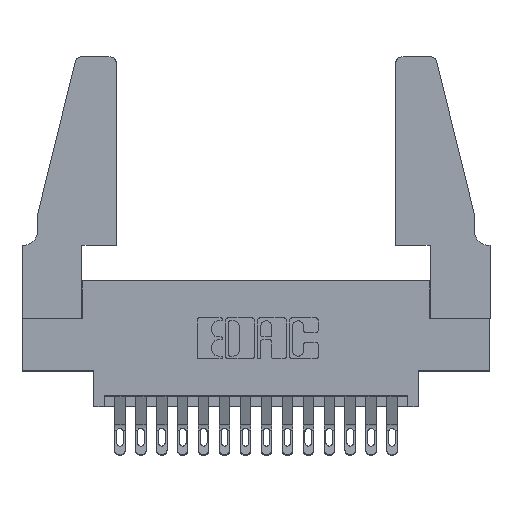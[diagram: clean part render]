
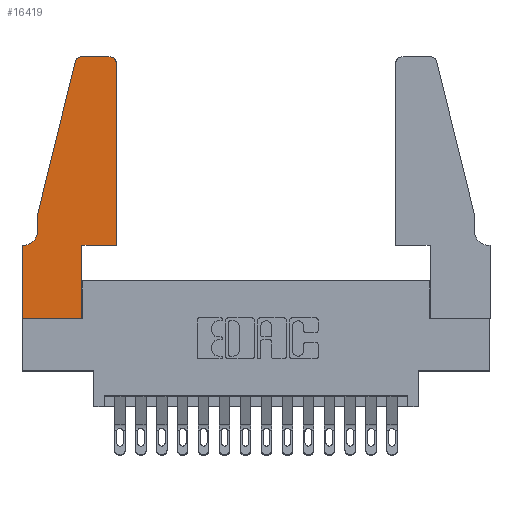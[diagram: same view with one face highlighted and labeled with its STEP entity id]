
A CAD part, top view. The second image highlights one B-rep face of the part: STEP entity #16419.
In plain terms, the highlighted planar face has unit normal (0, 0, 1).
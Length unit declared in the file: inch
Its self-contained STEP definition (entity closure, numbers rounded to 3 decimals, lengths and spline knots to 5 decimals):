
#64 = EDGE_CURVE ( 'NONE', #8364, #5197, #8122, .T. ) ;
#218 = CARTESIAN_POINT ( 'NONE',  ( 0.0755, 0.5, 0.37 ) ) ;
#368 = CARTESIAN_POINT ( 'NONE',  ( 0.25487, 1.22718, 0.37 ) ) ;
#1023 = DIRECTION ( 'NONE',  ( -1., 0., 0. ) ) ;
#1096 = CARTESIAN_POINT ( 'NONE',  ( 0.2865, 0.35, 0.37 ) ) ;
#1131 = EDGE_LOOP ( 'NONE', ( #15347, #12621, #10031, #10577, #16585, #2227, #10651, #14992, #3047, #8182, #17303, #7602 ) ) ;
#1283 = EDGE_CURVE ( 'NONE', #11010, #6689, #6015, .T. ) ;
#1339 = DIRECTION ( 'NONE',  ( -1., 0., 0. ) ) ;
#1574 = LINE ( 'NONE', #13921, #7477 ) ;
#2095 = CARTESIAN_POINT ( 'NONE',  ( 0.4205, 1.25, 0.37 ) ) ;
#2147 = CARTESIAN_POINT ( 'NONE',  ( 0.284, 1.25, 0.37 ) ) ;
#2157 = VECTOR ( 'NONE', #5187, 39.37008 ) ;
#2227 = ORIENTED_EDGE ( 'NONE', *, *, #13853, .T. ) ;
#2313 = DIRECTION ( 'NONE',  ( 0., 0., -1. ) ) ;
#2336 = DIRECTION ( 'NONE',  ( 1., 0., 0. ) ) ;
#2462 = DIRECTION ( 'NONE',  ( 0., 0., 1. ) ) ;
#2578 = DIRECTION ( 'NONE',  ( 1., 0., 0. ) ) ;
#2590 = CARTESIAN_POINT ( 'NONE',  ( 0.0755, 0.35, 0.37 ) ) ;
#3047 = ORIENTED_EDGE ( 'NONE', *, *, #3254, .T. ) ;
#3254 = EDGE_CURVE ( 'NONE', #6689, #9823, #7439, .T. ) ;
#3408 = DIRECTION ( 'NONE',  ( 0., -1., 0. ) ) ;
#3450 = LINE ( 'NONE', #3988, #16875 ) ;
#3749 = CARTESIAN_POINT ( 'NONE',  ( 0.4205, 1.22, 0.37 ) ) ;
#3792 = CARTESIAN_POINT ( 'NONE',  ( 0., 0., 0.37 ) ) ;
#3881 = DIRECTION ( 'NONE',  ( 1., 0., 0. ) ) ;
#3988 = CARTESIAN_POINT ( 'NONE',  ( 0.4505, 0.35, 0.37 ) ) ;
#4325 = LINE ( 'NONE', #218, #5160 ) ;
#5160 = VECTOR ( 'NONE', #15059, 39.37008 ) ;
#5187 = DIRECTION ( 'NONE',  ( 0., 1., 0. ) ) ;
#5197 = VERTEX_POINT ( 'NONE', #2147 ) ;
#5293 = VERTEX_POINT ( 'NONE', #8974 ) ;
#5543 = CARTESIAN_POINT ( 'NONE',  ( 0.0755, 0.5, 0.37 ) ) ;
#5597 = CARTESIAN_POINT ( 'NONE',  ( 0., 0.35, 0.37 ) ) ;
#5702 = VERTEX_POINT ( 'NONE', #12564 ) ;
#6015 = LINE ( 'NONE', #3792, #12689 ) ;
#6244 = VERTEX_POINT ( 'NONE', #16825 ) ;
#6287 = VECTOR ( 'NONE', #6887, 39.37008 ) ;
#6451 = CARTESIAN_POINT ( 'NONE',  ( 0., 0., 0.37 ) ) ;
#6472 = DIRECTION ( 'NONE',  ( 1., 0., 0. ) ) ;
#6506 = EDGE_CURVE ( 'NONE', #5293, #10681, #4325, .T. ) ;
#6513 = DIRECTION ( 'NONE',  ( 0., 0., 1. ) ) ;
#6689 = VERTEX_POINT ( 'NONE', #16376 ) ;
#6848 = EDGE_CURVE ( 'NONE', #5197, #8220, #9554, .T. ) ;
#6887 = DIRECTION ( 'NONE',  ( -0.239, -0.971, 0. ) ) ;
#7439 = LINE ( 'NONE', #13198, #2157 ) ;
#7462 = LINE ( 'NONE', #2590, #13279 ) ;
#7477 = VECTOR ( 'NONE', #16739, 39.37008 ) ;
#7592 = AXIS2_PLACEMENT_3D ( 'NONE', #3749, #6513, #2578 ) ;
#7602 = ORIENTED_EDGE ( 'NONE', *, *, #15196, .T. ) ;
#8122 = LINE ( 'NONE', #12547, #12719 ) ;
#8182 = ORIENTED_EDGE ( 'NONE', *, *, #13823, .T. ) ;
#8220 = VERTEX_POINT ( 'NONE', #368 ) ;
#8364 = VERTEX_POINT ( 'NONE', #2095 ) ;
#8600 = DIRECTION ( 'NONE',  ( -1., 0., 0. ) ) ;
#8974 = CARTESIAN_POINT ( 'NONE',  ( 0.0755, 0.5, 0.37 ) ) ;
#9554 = CIRCLE ( 'NONE', #12307, 0.03 ) ;
#9823 = VERTEX_POINT ( 'NONE', #1096 ) ;
#9841 = LINE ( 'NONE', #5543, #6287 ) ;
#9876 = LINE ( 'NONE', #15602, #12784 ) ;
#10031 = ORIENTED_EDGE ( 'NONE', *, *, #11094, .T. ) ;
#10458 = PLANE ( 'NONE',  #10833 ) ;
#10489 = CARTESIAN_POINT ( 'NONE',  ( 0.284, 1.22, 0.37 ) ) ;
#10577 = ORIENTED_EDGE ( 'NONE', *, *, #6506, .T. ) ;
#10599 = AXIS2_PLACEMENT_3D ( 'NONE', #17081, #2313, #1023 ) ;
#10651 = ORIENTED_EDGE ( 'NONE', *, *, #10788, .T. ) ;
#10681 = VERTEX_POINT ( 'NONE', #13841 ) ;
#10788 = EDGE_CURVE ( 'NONE', #13361, #11010, #9876, .T. ) ;
#10833 = AXIS2_PLACEMENT_3D ( 'NONE', #14497, #17253, #6472 ) ;
#11010 = VERTEX_POINT ( 'NONE', #6451 ) ;
#11094 = EDGE_CURVE ( 'NONE', #8220, #5293, #9841, .T. ) ;
#11358 = CARTESIAN_POINT ( 'NONE',  ( 0.0055, 0.35, 0.37 ) ) ;
#11422 = CIRCLE ( 'NONE', #10599, 0.07 ) ;
#11590 = CIRCLE ( 'NONE', #7592, 0.03 ) ;
#11815 = DIRECTION ( 'NONE',  ( 1., 0., 0. ) ) ;
#12307 = AXIS2_PLACEMENT_3D ( 'NONE', #10489, #2462, #11815 ) ;
#12547 = CARTESIAN_POINT ( 'NONE',  ( 0.2605, 1.25, 0.37 ) ) ;
#12564 = CARTESIAN_POINT ( 'NONE',  ( 0.4505, 0.35, 0.37 ) ) ;
#12621 = ORIENTED_EDGE ( 'NONE', *, *, #6848, .T. ) ;
#12689 = VECTOR ( 'NONE', #2336, 39.37008 ) ;
#12719 = VECTOR ( 'NONE', #8600, 39.37008 ) ;
#12784 = VECTOR ( 'NONE', #3408, 39.37008 ) ;
#13198 = CARTESIAN_POINT ( 'NONE',  ( 0.2865, 0.35, 0.37 ) ) ;
#13279 = VECTOR ( 'NONE', #1339, 39.37008 ) ;
#13361 = VERTEX_POINT ( 'NONE', #5597 ) ;
#13506 = EDGE_CURVE ( 'NONE', #5702, #6244, #1574, .T. ) ;
#13823 = EDGE_CURVE ( 'NONE', #9823, #5702, #3450, .T. ) ;
#13841 = CARTESIAN_POINT ( 'NONE',  ( 0.0755, 0.42, 0.37 ) ) ;
#13853 = EDGE_CURVE ( 'NONE', #15669, #13361, #7462, .T. ) ;
#13921 = CARTESIAN_POINT ( 'NONE',  ( 0.4505, 0.35, 0.37 ) ) ;
#14497 = CARTESIAN_POINT ( 'NONE',  ( 0., 0.35, 0.37 ) ) ;
#14501 = FACE_OUTER_BOUND ( 'NONE', #1131, .T. ) ;
#14503 = EDGE_CURVE ( 'NONE', #10681, #15669, #11422, .T. ) ;
#14992 = ORIENTED_EDGE ( 'NONE', *, *, #1283, .T. ) ;
#15059 = DIRECTION ( 'NONE',  ( 0., -1., 0. ) ) ;
#15196 = EDGE_CURVE ( 'NONE', #6244, #8364, #11590, .T. ) ;
#15347 = ORIENTED_EDGE ( 'NONE', *, *, #64, .T. ) ;
#15602 = CARTESIAN_POINT ( 'NONE',  ( 0., 0., 0.37 ) ) ;
#15669 = VERTEX_POINT ( 'NONE', #11358 ) ;
#16376 = CARTESIAN_POINT ( 'NONE',  ( 0.2865, 0., 0.37 ) ) ;
#16419 = ADVANCED_FACE ( 'NONE', ( #14501 ), #10458, .T. ) ;
#16585 = ORIENTED_EDGE ( 'NONE', *, *, #14503, .T. ) ;
#16739 = DIRECTION ( 'NONE',  ( 0., 1., 0. ) ) ;
#16825 = CARTESIAN_POINT ( 'NONE',  ( 0.4505, 1.22, 0.37 ) ) ;
#16875 = VECTOR ( 'NONE', #3881, 39.37008 ) ;
#17081 = CARTESIAN_POINT ( 'NONE',  ( 0.0055, 0.42, 0.37 ) ) ;
#17253 = DIRECTION ( 'NONE',  ( 0., 0., 1. ) ) ;
#17303 = ORIENTED_EDGE ( 'NONE', *, *, #13506, .T. ) ;
